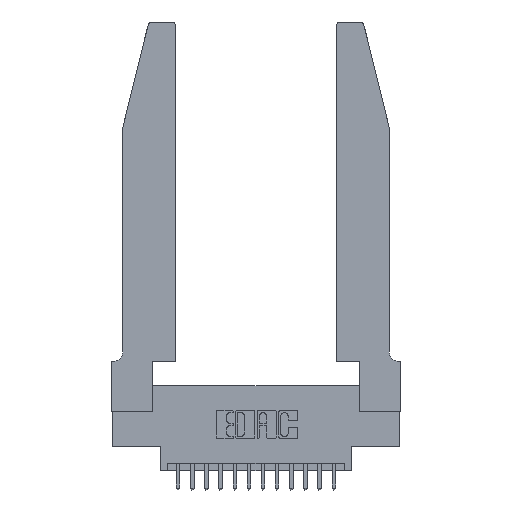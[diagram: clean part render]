
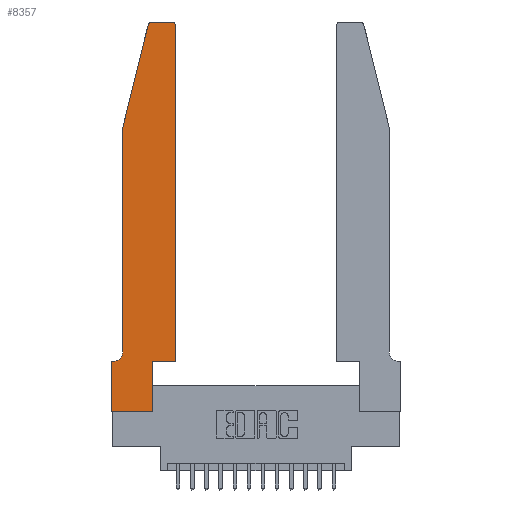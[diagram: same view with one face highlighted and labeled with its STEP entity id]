
A CAD part, top view. The second image highlights one B-rep face of the part: STEP entity #8357.
In plain terms, the highlighted planar face has unit normal (0, 0, 1).
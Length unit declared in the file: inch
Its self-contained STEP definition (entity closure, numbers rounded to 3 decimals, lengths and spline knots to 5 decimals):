
#36 = CARTESIAN_POINT ( 'NONE',  ( 0., 0.35, 0.37 ) ) ;
#228 = ORIENTED_EDGE ( 'NONE', *, *, #11652, .T. ) ;
#314 = CIRCLE ( 'NONE', #16353, 0.03 ) ;
#792 = DIRECTION ( 'NONE',  ( 0., 0., 1. ) ) ;
#918 = DIRECTION ( 'NONE',  ( 0., 0., -1. ) ) ;
#1039 = CARTESIAN_POINT ( 'NONE',  ( 0.0055, 0.35, 0.37 ) ) ;
#1403 = AXIS2_PLACEMENT_3D ( 'NONE', #11717, #4839, #6238 ) ;
#1635 = ORIENTED_EDGE ( 'NONE', *, *, #17735, .T. ) ;
#1642 = ORIENTED_EDGE ( 'NONE', *, *, #12745, .T. ) ;
#1883 = ORIENTED_EDGE ( 'NONE', *, *, #10846, .T. ) ;
#2040 = VERTEX_POINT ( 'NONE', #5026 ) ;
#2156 = DIRECTION ( 'NONE',  ( 1., 0., 0. ) ) ;
#2287 = CARTESIAN_POINT ( 'NONE',  ( 0.4205, 2.72, 0.37 ) ) ;
#2657 = CARTESIAN_POINT ( 'NONE',  ( 0., 0., 0.37 ) ) ;
#2678 = EDGE_CURVE ( 'NONE', #14789, #6963, #4027, .T. ) ;
#3052 = DIRECTION ( 'NONE',  ( 0., -1., 0. ) ) ;
#3526 = CARTESIAN_POINT ( 'NONE',  ( 0.284, 2.72, 0.37 ) ) ;
#3594 = EDGE_LOOP ( 'NONE', ( #1642, #1635, #7726, #5081, #13735, #14878, #228, #13562, #5165, #6511, #4610, #1883 ) ) ;
#3884 = CARTESIAN_POINT ( 'NONE',  ( 0.25487, 2.72718, 0.37 ) ) ;
#3930 = DIRECTION ( 'NONE',  ( -1., 0., 0. ) ) ;
#4027 = LINE ( 'NONE', #11499, #15999 ) ;
#4046 = CIRCLE ( 'NONE', #9524, 0.07 ) ;
#4610 = ORIENTED_EDGE ( 'NONE', *, *, #10756, .T. ) ;
#4634 = DIRECTION ( 'NONE',  ( 0., 1., 0. ) ) ;
#4839 = DIRECTION ( 'NONE',  ( 0., 0., 1. ) ) ;
#4915 = VECTOR ( 'NONE', #3930, 39.37008 ) ;
#4978 = DIRECTION ( 'NONE',  ( 0., 0., 1. ) ) ;
#5026 = CARTESIAN_POINT ( 'NONE',  ( 0.4505, 2.72, 0.37 ) ) ;
#5079 = DIRECTION ( 'NONE',  ( -1., 0., 0. ) ) ;
#5081 = ORIENTED_EDGE ( 'NONE', *, *, #2678, .T. ) ;
#5165 = ORIENTED_EDGE ( 'NONE', *, *, #9754, .T. ) ;
#5206 = DIRECTION ( 'NONE',  ( -1., 0., 0. ) ) ;
#5355 = FACE_OUTER_BOUND ( 'NONE', #3594, .T. ) ;
#5804 = LINE ( 'NONE', #13113, #12462 ) ;
#6223 = CARTESIAN_POINT ( 'NONE',  ( 0.0755, 2., 0.37 ) ) ;
#6238 = DIRECTION ( 'NONE',  ( 1., 0., 0. ) ) ;
#6511 = ORIENTED_EDGE ( 'NONE', *, *, #8765, .T. ) ;
#6832 = DIRECTION ( 'NONE',  ( 0., -1., 0. ) ) ;
#6941 = VECTOR ( 'NONE', #10466, 39.37008 ) ;
#6963 = VERTEX_POINT ( 'NONE', #7589 ) ;
#7331 = PLANE ( 'NONE',  #1403 ) ;
#7420 = VECTOR ( 'NONE', #6832, 39.37008 ) ;
#7589 = CARTESIAN_POINT ( 'NONE',  ( 0.0755, 0.42, 0.37 ) ) ;
#7726 = ORIENTED_EDGE ( 'NONE', *, *, #9776, .T. ) ;
#7838 = CARTESIAN_POINT ( 'NONE',  ( 0.0055, 0.42, 0.37 ) ) ;
#7971 = VERTEX_POINT ( 'NONE', #2657 ) ;
#8297 = VECTOR ( 'NONE', #10192, 39.37008 ) ;
#8357 = ADVANCED_FACE ( 'NONE', ( #5355 ), #7331, .T. ) ;
#8401 = CARTESIAN_POINT ( 'NONE',  ( 0.284, 2.75, 0.37 ) ) ;
#8455 = VERTEX_POINT ( 'NONE', #1039 ) ;
#8516 = CARTESIAN_POINT ( 'NONE',  ( 0., 0., 0.37 ) ) ;
#8765 = EDGE_CURVE ( 'NONE', #13412, #11886, #16254, .T. ) ;
#9445 = EDGE_CURVE ( 'NONE', #6963, #8455, #4046, .T. ) ;
#9524 = AXIS2_PLACEMENT_3D ( 'NONE', #7838, #918, #5079 ) ;
#9754 = EDGE_CURVE ( 'NONE', #16012, #13412, #17556, .T. ) ;
#9776 = EDGE_CURVE ( 'NONE', #13901, #14789, #12246, .T. ) ;
#10004 = CARTESIAN_POINT ( 'NONE',  ( 0.4505, 0.35, 0.37 ) ) ;
#10192 = DIRECTION ( 'NONE',  ( 1., 0., 0. ) ) ;
#10466 = DIRECTION ( 'NONE',  ( -0.239, -0.971, 0. ) ) ;
#10756 = EDGE_CURVE ( 'NONE', #11886, #2040, #5804, .T. ) ;
#10821 = LINE ( 'NONE', #15310, #17688 ) ;
#10846 = EDGE_CURVE ( 'NONE', #2040, #17230, #15339, .T. ) ;
#11499 = CARTESIAN_POINT ( 'NONE',  ( 0.0755, 2., 0.37 ) ) ;
#11584 = CARTESIAN_POINT ( 'NONE',  ( 0.4505, 0.35, 0.37 ) ) ;
#11592 = CARTESIAN_POINT ( 'NONE',  ( 0.2865, 0.35, 0.37 ) ) ;
#11652 = EDGE_CURVE ( 'NONE', #14131, #7971, #13852, .T. ) ;
#11717 = CARTESIAN_POINT ( 'NONE',  ( 0., 0.35, 0.37 ) ) ;
#11886 = VERTEX_POINT ( 'NONE', #11584 ) ;
#12056 = LINE ( 'NONE', #8516, #14714 ) ;
#12246 = LINE ( 'NONE', #6223, #6941 ) ;
#12380 = CARTESIAN_POINT ( 'NONE',  ( 0.4205, 2.75, 0.37 ) ) ;
#12462 = VECTOR ( 'NONE', #4634, 39.37008 ) ;
#12745 = EDGE_CURVE ( 'NONE', #17230, #18026, #18234, .T. ) ;
#13113 = CARTESIAN_POINT ( 'NONE',  ( 0.4505, 0.35, 0.37 ) ) ;
#13412 = VERTEX_POINT ( 'NONE', #11592 ) ;
#13562 = ORIENTED_EDGE ( 'NONE', *, *, #18006, .T. ) ;
#13735 = ORIENTED_EDGE ( 'NONE', *, *, #9445, .T. ) ;
#13852 = LINE ( 'NONE', #16745, #7420 ) ;
#13901 = VERTEX_POINT ( 'NONE', #3884 ) ;
#14131 = VERTEX_POINT ( 'NONE', #36 ) ;
#14166 = DIRECTION ( 'NONE',  ( 1., 0., 0. ) ) ;
#14714 = VECTOR ( 'NONE', #14166, 39.37008 ) ;
#14789 = VERTEX_POINT ( 'NONE', #15884 ) ;
#14878 = ORIENTED_EDGE ( 'NONE', *, *, #15138, .T. ) ;
#15138 = EDGE_CURVE ( 'NONE', #8455, #14131, #10821, .T. ) ;
#15271 = CARTESIAN_POINT ( 'NONE',  ( 0.2605, 2.75, 0.37 ) ) ;
#15310 = CARTESIAN_POINT ( 'NONE',  ( 0.0755, 0.35, 0.37 ) ) ;
#15339 = CIRCLE ( 'NONE', #16052, 0.03 ) ;
#15487 = CARTESIAN_POINT ( 'NONE',  ( 0.2865, 0., 0.37 ) ) ;
#15572 = VECTOR ( 'NONE', #16036, 39.37008 ) ;
#15884 = CARTESIAN_POINT ( 'NONE',  ( 0.0755, 2., 0.37 ) ) ;
#15919 = CARTESIAN_POINT ( 'NONE',  ( 0.2865, 0.35, 0.37 ) ) ;
#15999 = VECTOR ( 'NONE', #3052, 39.37008 ) ;
#16012 = VERTEX_POINT ( 'NONE', #15487 ) ;
#16036 = DIRECTION ( 'NONE',  ( 0., 1., 0. ) ) ;
#16052 = AXIS2_PLACEMENT_3D ( 'NONE', #2287, #792, #2156 ) ;
#16254 = LINE ( 'NONE', #10004, #8297 ) ;
#16353 = AXIS2_PLACEMENT_3D ( 'NONE', #3526, #4978, #17689 ) ;
#16745 = CARTESIAN_POINT ( 'NONE',  ( 0., 0., 0.37 ) ) ;
#17230 = VERTEX_POINT ( 'NONE', #12380 ) ;
#17556 = LINE ( 'NONE', #15919, #15572 ) ;
#17688 = VECTOR ( 'NONE', #5206, 39.37008 ) ;
#17689 = DIRECTION ( 'NONE',  ( 1., 0., 0. ) ) ;
#17735 = EDGE_CURVE ( 'NONE', #18026, #13901, #314, .T. ) ;
#18006 = EDGE_CURVE ( 'NONE', #7971, #16012, #12056, .T. ) ;
#18026 = VERTEX_POINT ( 'NONE', #8401 ) ;
#18234 = LINE ( 'NONE', #15271, #4915 ) ;
